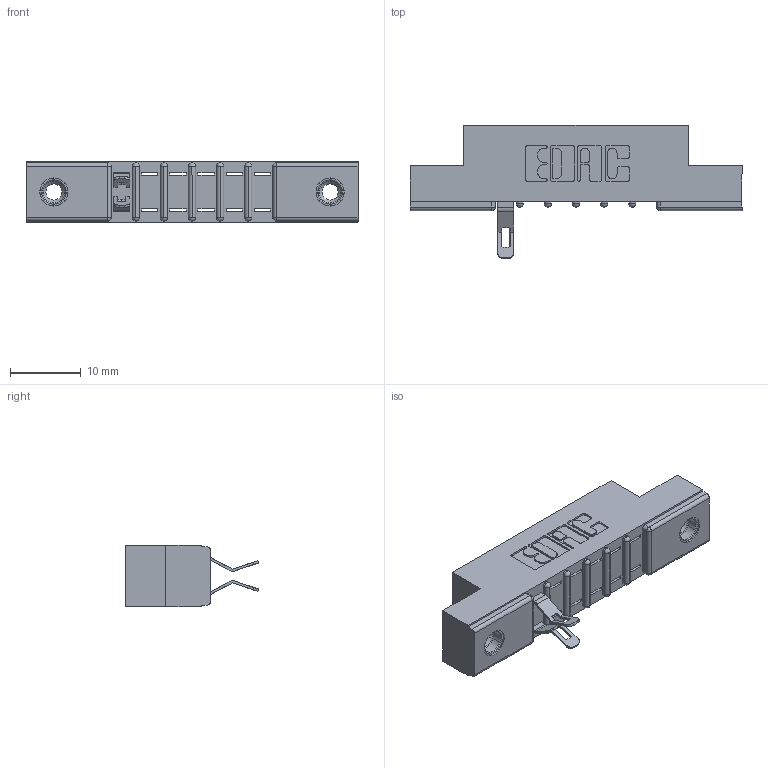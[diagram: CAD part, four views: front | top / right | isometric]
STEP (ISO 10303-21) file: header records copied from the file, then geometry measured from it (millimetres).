
FILE_DESCRIPTION (( 'STEP AP203' ), '1' );
FILE_NAME ('357-012-555-208.STEP', '2018-08-07T22:14:14', ( '' ), ( '' ), 'SwSTEP 2.0', 'SolidWorks 2016', '' );
FILE_SCHEMA (( 'CONFIG_CONTROL_DESIGN' ));
Length unit declared in the file: inch
Products named in the file (4): 345-250-001_345-250-003-102; 357-012-555-208; 307 Part_.156 Dia Mounting Holes; 307-290-001_555
Assembly tree (5 placements, depth 2):
  357-012-555-208
    307 Part_.156 Dia Mounting Holes
    307-290-001_555  x2
    345-250-001_345-250-003-102  x2
Bounding box: 46.79 x 18.75 x 8.71 mm (x, y, z)
Volume: 2932.1 mm3; surface area: 3634.4 mm2
Topology: 5 solids, 5 shells, 407 faces, 1141 edges, 730 vertices
Faces by surface type: plane 230, cylinder 147, sphere 14, cone 12, torus 4
Entity records: 11176 total; most frequent: CARTESIAN_POINT 1871, ORIENTED_EDGE 1856, DIRECTION 1854, EDGE_CURVE 928, LINE 684, VECTOR 684, VERTEX_POINT 602, AXIS2_PLACEMENT_3D 585
